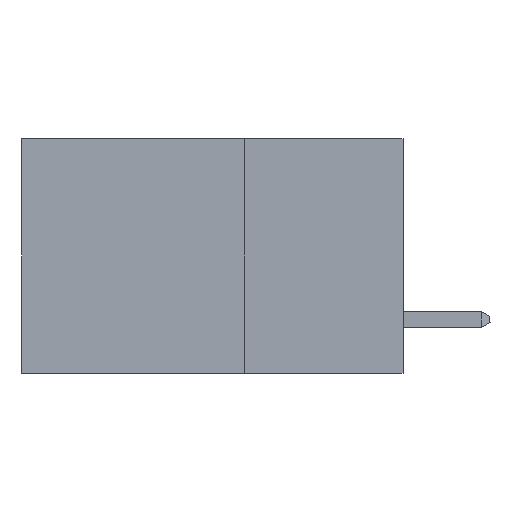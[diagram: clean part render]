
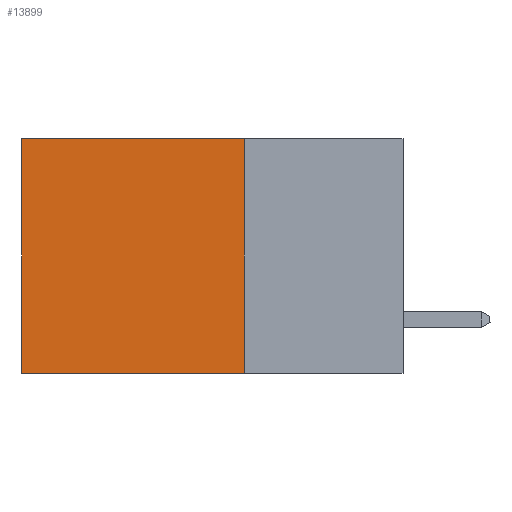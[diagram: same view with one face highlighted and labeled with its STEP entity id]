
A CAD part, left-side view. The second image highlights one B-rep face of the part: STEP entity #13899.
In plain terms, the highlighted planar face has unit normal (-1, 0, 0).
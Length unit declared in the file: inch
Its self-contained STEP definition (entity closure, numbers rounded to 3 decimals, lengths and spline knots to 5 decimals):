
#62 = ORIENTED_EDGE ( 'NONE', *, *, #3097, .F. ) ;
#453 = AXIS2_PLACEMENT_3D ( 'NONE', #3485, #6174, #11059 ) ;
#893 = LINE ( 'NONE', #5463, #15257 ) ;
#1122 = LINE ( 'NONE', #14073, #11663 ) ;
#2178 = DIRECTION ( 'NONE',  ( 0., 0., -1. ) ) ;
#2371 = VERTEX_POINT ( 'NONE', #11307 ) ;
#2711 = VECTOR ( 'NONE', #2178, 39.37008 ) ;
#2798 = CARTESIAN_POINT ( 'NONE',  ( 0.2875, 0.25, 0. ) ) ;
#3097 = EDGE_CURVE ( 'NONE', #15633, #2371, #1122, .T. ) ;
#3481 = CARTESIAN_POINT ( 'NONE',  ( 0.2875, 0.25, 0. ) ) ;
#3485 = CARTESIAN_POINT ( 'NONE',  ( 0.2875, 0.25, 0. ) ) ;
#3976 = ORIENTED_EDGE ( 'NONE', *, *, #10309, .T. ) ;
#4301 = VERTEX_POINT ( 'NONE', #3481 ) ;
#4495 = EDGE_CURVE ( 'NONE', #4301, #15633, #15023, .T. ) ;
#5463 = CARTESIAN_POINT ( 'NONE',  ( 0.2875, 0.25, 0. ) ) ;
#5567 = LINE ( 'NONE', #13724, #2711 ) ;
#6174 = DIRECTION ( 'NONE',  ( 1., 0., 0. ) ) ;
#6544 = DIRECTION ( 'NONE',  ( 0., 1., 0. ) ) ;
#8097 = CARTESIAN_POINT ( 'NONE',  ( 0.2875, 0.6, 0. ) ) ;
#8213 = EDGE_LOOP ( 'NONE', ( #15085, #62, #12512, #3976 ) ) ;
#9191 = VERTEX_POINT ( 'NONE', #8097 ) ;
#10309 = EDGE_CURVE ( 'NONE', #4301, #9191, #893, .T. ) ;
#10609 = EDGE_CURVE ( 'NONE', #9191, #2371, #5567, .T. ) ;
#11059 = DIRECTION ( 'NONE',  ( 0., 0., -1. ) ) ;
#11307 = CARTESIAN_POINT ( 'NONE',  ( 0.2875, 0.6, -0.37 ) ) ;
#11663 = VECTOR ( 'NONE', #6544, 39.37008 ) ;
#11854 = DIRECTION ( 'NONE',  ( 0., 0., -1. ) ) ;
#12512 = ORIENTED_EDGE ( 'NONE', *, *, #4495, .F. ) ;
#13432 = VECTOR ( 'NONE', #11854, 39.37008 ) ;
#13724 = CARTESIAN_POINT ( 'NONE',  ( 0.2875, 0.6, 0. ) ) ;
#13899 = ADVANCED_FACE ( 'NONE', ( #16763 ), #15124, .F. ) ;
#14071 = CARTESIAN_POINT ( 'NONE',  ( 0.2875, 0.25, -0.37 ) ) ;
#14073 = CARTESIAN_POINT ( 'NONE',  ( 0.2875, 0.25, -0.37 ) ) ;
#14312 = DIRECTION ( 'NONE',  ( 0., 1., 0. ) ) ;
#15023 = LINE ( 'NONE', #2798, #13432 ) ;
#15085 = ORIENTED_EDGE ( 'NONE', *, *, #10609, .T. ) ;
#15124 = PLANE ( 'NONE',  #453 ) ;
#15257 = VECTOR ( 'NONE', #14312, 39.37008 ) ;
#15633 = VERTEX_POINT ( 'NONE', #14071 ) ;
#16763 = FACE_OUTER_BOUND ( 'NONE', #8213, .T. ) ;
